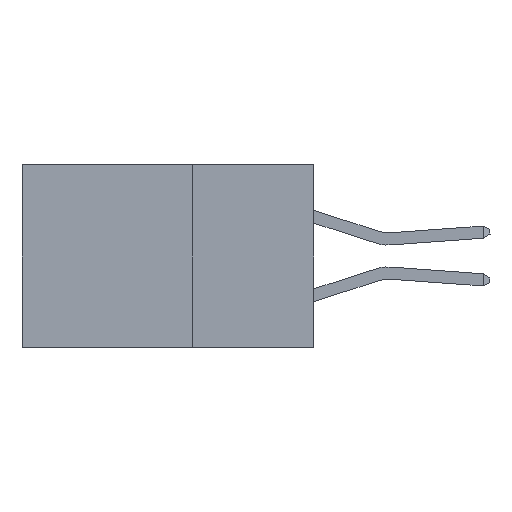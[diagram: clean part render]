
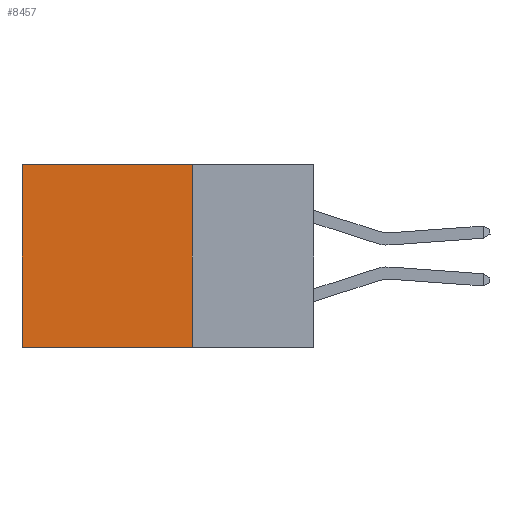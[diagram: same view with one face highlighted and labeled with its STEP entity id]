
A CAD part, left-side view. The second image highlights one B-rep face of the part: STEP entity #8457.
In plain terms, the highlighted planar face has unit normal (-1, 0, 0).
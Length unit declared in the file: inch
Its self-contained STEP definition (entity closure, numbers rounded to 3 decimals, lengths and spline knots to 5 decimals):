
#72 = EDGE_CURVE ( 'NONE', #6931, #2428, #12203, .T. ) ;
#487 = LINE ( 'NONE', #13433, #12851 ) ;
#1171 = VECTOR ( 'NONE', #1762, 39.37008 ) ;
#1762 = DIRECTION ( 'NONE',  ( 0., 0., -1. ) ) ;
#2069 = ORIENTED_EDGE ( 'NONE', *, *, #72, .T. ) ;
#2428 = VERTEX_POINT ( 'NONE', #7504 ) ;
#3049 = CARTESIAN_POINT ( 'NONE',  ( 0.2875, 0.25, -0.375 ) ) ;
#3465 = LINE ( 'NONE', #10204, #13886 ) ;
#3488 = ORIENTED_EDGE ( 'NONE', *, *, #6790, .F. ) ;
#4614 = DIRECTION ( 'NONE',  ( 0., 0., -1. ) ) ;
#5186 = ORIENTED_EDGE ( 'NONE', *, *, #8760, .T. ) ;
#5645 = CARTESIAN_POINT ( 'NONE',  ( 0.2875, 0.25, -0.375 ) ) ;
#5727 = DIRECTION ( 'NONE',  ( 1., 0., 0. ) ) ;
#6785 = PLANE ( 'NONE',  #10687 ) ;
#6790 = EDGE_CURVE ( 'NONE', #12637, #13088, #3465, .T. ) ;
#6931 = VERTEX_POINT ( 'NONE', #14643 ) ;
#6943 = DIRECTION ( 'NONE',  ( 0., 0., -1. ) ) ;
#7464 = EDGE_CURVE ( 'NONE', #13088, #2428, #7818, .T. ) ;
#7504 = CARTESIAN_POINT ( 'NONE',  ( 0.2875, 0.6, -0.375 ) ) ;
#7756 = DIRECTION ( 'NONE',  ( 0., 1., 0. ) ) ;
#7818 = LINE ( 'NONE', #3049, #10715 ) ;
#8457 = ADVANCED_FACE ( 'NONE', ( #9286 ), #6785, .F. ) ;
#8760 = EDGE_CURVE ( 'NONE', #12637, #6931, #487, .T. ) ;
#8805 = ORIENTED_EDGE ( 'NONE', *, *, #7464, .F. ) ;
#9286 = FACE_OUTER_BOUND ( 'NONE', #9814, .T. ) ;
#9814 = EDGE_LOOP ( 'NONE', ( #2069, #8805, #3488, #5186 ) ) ;
#10204 = CARTESIAN_POINT ( 'NONE',  ( 0.2875, 0.25, -0.375 ) ) ;
#10687 = AXIS2_PLACEMENT_3D ( 'NONE', #5645, #5727, #6943 ) ;
#10715 = VECTOR ( 'NONE', #7756, 39.37008 ) ;
#12203 = LINE ( 'NONE', #14560, #1171 ) ;
#12229 = CARTESIAN_POINT ( 'NONE',  ( 0.2875, 0.25, -0.375 ) ) ;
#12253 = CARTESIAN_POINT ( 'NONE',  ( 0.2875, 0.25, 0. ) ) ;
#12637 = VERTEX_POINT ( 'NONE', #12253 ) ;
#12851 = VECTOR ( 'NONE', #13122, 39.37008 ) ;
#13088 = VERTEX_POINT ( 'NONE', #12229 ) ;
#13122 = DIRECTION ( 'NONE',  ( 0., 1., 0. ) ) ;
#13433 = CARTESIAN_POINT ( 'NONE',  ( 0.2875, 0.25, 0. ) ) ;
#13886 = VECTOR ( 'NONE', #4614, 39.37008 ) ;
#14560 = CARTESIAN_POINT ( 'NONE',  ( 0.2875, 0.6, -0.375 ) ) ;
#14643 = CARTESIAN_POINT ( 'NONE',  ( 0.2875, 0.6, 0. ) ) ;
